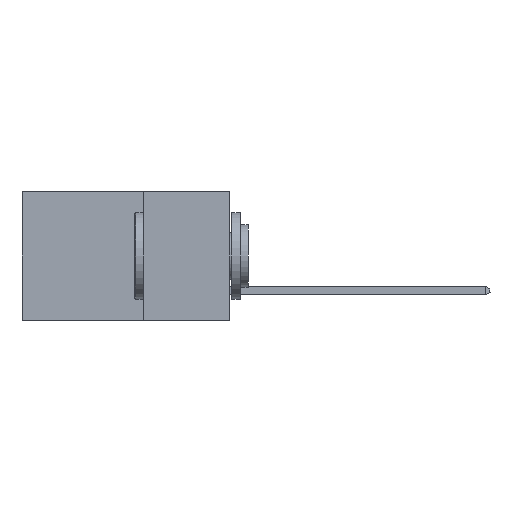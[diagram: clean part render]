
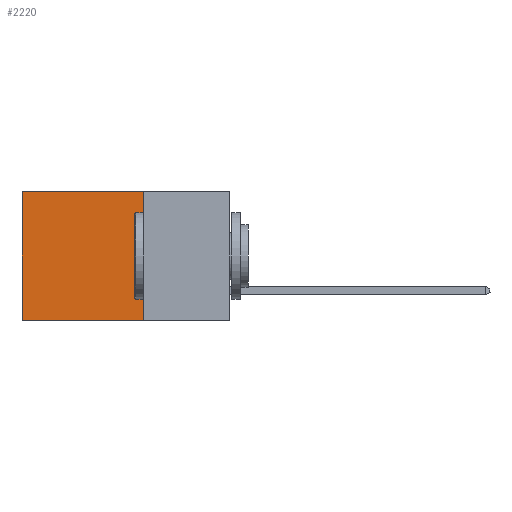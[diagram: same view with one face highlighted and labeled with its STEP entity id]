
A CAD part, left-side view. The second image highlights one B-rep face of the part: STEP entity #2220.
In plain terms, the highlighted planar face has unit normal (-1, 0, 0).
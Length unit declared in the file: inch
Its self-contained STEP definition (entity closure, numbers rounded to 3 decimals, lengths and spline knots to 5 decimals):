
#952 = VERTEX_POINT ( 'NONE', #8710 ) ;
#961 = VERTEX_POINT ( 'NONE', #1201 ) ;
#1094 = DIRECTION ( 'NONE',  ( 0., 1., 0. ) ) ;
#1149 = PLANE ( 'NONE',  #8635 ) ;
#1201 = CARTESIAN_POINT ( 'NONE',  ( 0.298, 0.6, -0.37 ) ) ;
#1426 = EDGE_CURVE ( 'NONE', #9182, #961, #3782, .T. ) ;
#1511 = EDGE_CURVE ( 'NONE', #1820, #9182, #4804, .T. ) ;
#1820 = VERTEX_POINT ( 'NONE', #8912 ) ;
#2216 = VECTOR ( 'NONE', #12030, 39.37008 ) ;
#2220 = ADVANCED_FACE ( 'NONE', ( #7444 ), #1149, .F. ) ;
#3782 = LINE ( 'NONE', #11634, #9071 ) ;
#3924 = ORIENTED_EDGE ( 'NONE', *, *, #1511, .T. ) ;
#4105 = VECTOR ( 'NONE', #1094, 39.37008 ) ;
#4163 = DIRECTION ( 'NONE',  ( 1., 0., 0. ) ) ;
#4588 = LINE ( 'NONE', #9234, #2216 ) ;
#4804 = LINE ( 'NONE', #8108, #11919 ) ;
#5203 = EDGE_CURVE ( 'NONE', #952, #961, #9849, .T. ) ;
#6030 = ORIENTED_EDGE ( 'NONE', *, *, #5203, .F. ) ;
#6061 = CARTESIAN_POINT ( 'NONE',  ( 0.298, 0.25, 0. ) ) ;
#6314 = ORIENTED_EDGE ( 'NONE', *, *, #9376, .F. ) ;
#6725 = CARTESIAN_POINT ( 'NONE',  ( 0.298, 0.25, -0.37 ) ) ;
#6974 = CARTESIAN_POINT ( 'NONE',  ( 0.298, 0.6, 0. ) ) ;
#7444 = FACE_OUTER_BOUND ( 'NONE', #7518, .T. ) ;
#7518 = EDGE_LOOP ( 'NONE', ( #10488, #6030, #6314, #3924 ) ) ;
#7881 = DIRECTION ( 'NONE',  ( 0., 0., -1. ) ) ;
#8108 = CARTESIAN_POINT ( 'NONE',  ( 0.298, 0.25, 0. ) ) ;
#8635 = AXIS2_PLACEMENT_3D ( 'NONE', #6061, #4163, #7881 ) ;
#8710 = CARTESIAN_POINT ( 'NONE',  ( 0.298, 0.25, -0.37 ) ) ;
#8912 = CARTESIAN_POINT ( 'NONE',  ( 0.298, 0.25, 0. ) ) ;
#9071 = VECTOR ( 'NONE', #10729, 39.37008 ) ;
#9182 = VERTEX_POINT ( 'NONE', #6974 ) ;
#9234 = CARTESIAN_POINT ( 'NONE',  ( 0.298, 0.25, 0. ) ) ;
#9376 = EDGE_CURVE ( 'NONE', #1820, #952, #4588, .T. ) ;
#9849 = LINE ( 'NONE', #6725, #4105 ) ;
#10488 = ORIENTED_EDGE ( 'NONE', *, *, #1426, .T. ) ;
#10729 = DIRECTION ( 'NONE',  ( 0., 0., -1. ) ) ;
#11634 = CARTESIAN_POINT ( 'NONE',  ( 0.298, 0.6, 0. ) ) ;
#11919 = VECTOR ( 'NONE', #11938, 39.37008 ) ;
#11938 = DIRECTION ( 'NONE',  ( 0., 1., 0. ) ) ;
#12030 = DIRECTION ( 'NONE',  ( 0., 0., -1. ) ) ;
